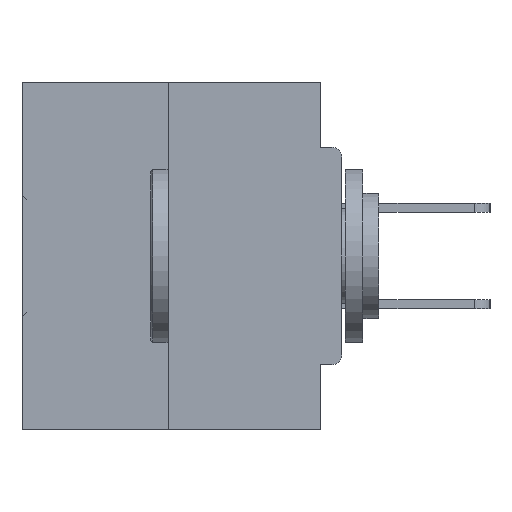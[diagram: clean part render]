
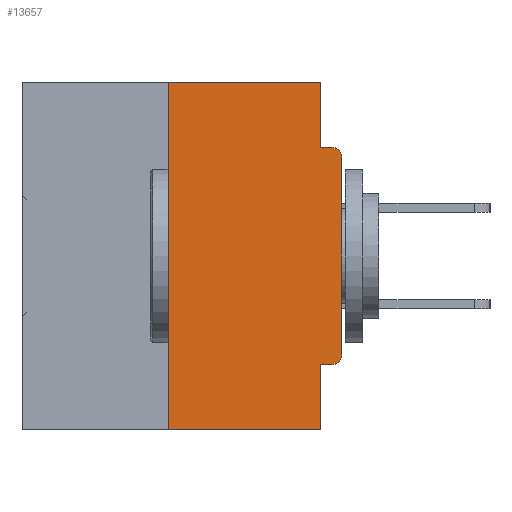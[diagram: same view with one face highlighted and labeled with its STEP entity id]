
A CAD part, left-side view. The second image highlights one B-rep face of the part: STEP entity #13657.
In plain terms, the highlighted planar face has unit normal (-1, 0, 0).
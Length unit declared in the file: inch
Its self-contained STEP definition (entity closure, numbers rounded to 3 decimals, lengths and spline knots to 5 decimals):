
#447 = CARTESIAN_POINT ( 'NONE',  ( 0., 0.015, -0.1085 ) ) ;
#537 = EDGE_CURVE ( 'NONE', #41187, #37084, #8913, .T. ) ;
#1069 = VECTOR ( 'NONE', #31670, 39.37008 ) ;
#1840 = CARTESIAN_POINT ( 'NONE',  ( 0., 0.031, -0.4065 ) ) ;
#3988 = CARTESIAN_POINT ( 'NONE',  ( 0., 0., -0.3915 ) ) ;
#4064 = VERTEX_POINT ( 'NONE', #1840 ) ;
#4535 = VECTOR ( 'NONE', #21475, 39.37008 ) ;
#4632 = CARTESIAN_POINT ( 'NONE',  ( 0., 0.031, 0. ) ) ;
#4937 = DIRECTION ( 'NONE',  ( 0., 0., -1. ) ) ;
#6304 = VERTEX_POINT ( 'NONE', #32371 ) ;
#6608 = ORIENTED_EDGE ( 'NONE', *, *, #36303, .T. ) ;
#6632 = AXIS2_PLACEMENT_3D ( 'NONE', #26175, #19660, #22784 ) ;
#6746 = DIRECTION ( 'NONE',  ( 0., -1., 0. ) ) ;
#7027 = VERTEX_POINT ( 'NONE', #24200 ) ;
#7271 = VECTOR ( 'NONE', #23623, 39.37008 ) ;
#7491 = DIRECTION ( 'NONE',  ( -1., 0., 0. ) ) ;
#7842 = LINE ( 'NONE', #17770, #4535 ) ;
#7940 = ORIENTED_EDGE ( 'NONE', *, *, #32972, .F. ) ;
#8913 = LINE ( 'NONE', #41056, #7271 ) ;
#9235 = VECTOR ( 'NONE', #4937, 39.37008 ) ;
#11164 = ORIENTED_EDGE ( 'NONE', *, *, #537, .F. ) ;
#11357 = EDGE_CURVE ( 'NONE', #4064, #7027, #14936, .T. ) ;
#12130 = LINE ( 'NONE', #26361, #39038 ) ;
#12963 = EDGE_CURVE ( 'NONE', #26523, #42302, #18642, .T. ) ;
#13657 = ADVANCED_FACE ( 'NONE', ( #19707 ), #43288, .F. ) ;
#13735 = CARTESIAN_POINT ( 'NONE',  ( 0., 0.031, 0. ) ) ;
#14194 = LINE ( 'NONE', #4632, #9235 ) ;
#14375 = CARTESIAN_POINT ( 'NONE',  ( 0., 0.46, -0.5 ) ) ;
#14936 = LINE ( 'NONE', #36313, #19318 ) ;
#15106 = ORIENTED_EDGE ( 'NONE', *, *, #38545, .F. ) ;
#15261 = DIRECTION ( 'NONE',  ( 0., 0., -1. ) ) ;
#16286 = EDGE_CURVE ( 'NONE', #37921, #42302, #22758, .T. ) ;
#16679 = ORIENTED_EDGE ( 'NONE', *, *, #24940, .F. ) ;
#17695 = CARTESIAN_POINT ( 'NONE',  ( 0., 0., -0.4065 ) ) ;
#17770 = CARTESIAN_POINT ( 'NONE',  ( 0., 0., 0. ) ) ;
#18613 = DIRECTION ( 'NONE',  ( 1., 0., 0. ) ) ;
#18642 = LINE ( 'NONE', #31029, #40022 ) ;
#18664 = EDGE_LOOP ( 'NONE', ( #11164, #15106, #6608, #20464, #7940, #38362, #26435, #30995, #33911, #16679 ) ) ;
#19185 = CIRCLE ( 'NONE', #6632, 0.015 ) ;
#19318 = VECTOR ( 'NONE', #15261, 39.37008 ) ;
#19660 = DIRECTION ( 'NONE',  ( -1., 0., 0. ) ) ;
#19707 = FACE_OUTER_BOUND ( 'NONE', #18664, .T. ) ;
#20464 = ORIENTED_EDGE ( 'NONE', *, *, #11357, .F. ) ;
#20651 = CARTESIAN_POINT ( 'NONE',  ( 0., 0.25, -0.5 ) ) ;
#21475 = DIRECTION ( 'NONE',  ( 0., 0., 1. ) ) ;
#22758 = CIRCLE ( 'NONE', #41384, 0.015 ) ;
#22784 = DIRECTION ( 'NONE',  ( 0., 0., -1. ) ) ;
#23623 = DIRECTION ( 'NONE',  ( 0., -1., 0. ) ) ;
#24200 = CARTESIAN_POINT ( 'NONE',  ( 0., 0.031, -0.5 ) ) ;
#24855 = DIRECTION ( 'NONE',  ( 0., -1., 0. ) ) ;
#24915 = DIRECTION ( 'NONE',  ( 0., 0., -1. ) ) ;
#24940 = EDGE_CURVE ( 'NONE', #37084, #26523, #14194, .T. ) ;
#25851 = CARTESIAN_POINT ( 'NONE',  ( 0., 0.46, 0. ) ) ;
#26175 = CARTESIAN_POINT ( 'NONE',  ( 0., 0.015, -0.3915 ) ) ;
#26361 = CARTESIAN_POINT ( 'NONE',  ( 0., 0.25, 0. ) ) ;
#26435 = ORIENTED_EDGE ( 'NONE', *, *, #36073, .T. ) ;
#26523 = VERTEX_POINT ( 'NONE', #44175 ) ;
#30957 = CARTESIAN_POINT ( 'NONE',  ( 0., 0.015, -0.0935 ) ) ;
#30995 = ORIENTED_EDGE ( 'NONE', *, *, #16286, .T. ) ;
#31007 = VERTEX_POINT ( 'NONE', #20651 ) ;
#31029 = CARTESIAN_POINT ( 'NONE',  ( 0., 0., -0.0935 ) ) ;
#31291 = LINE ( 'NONE', #17695, #1069 ) ;
#31670 = DIRECTION ( 'NONE',  ( 0., 1., 0. ) ) ;
#32371 = CARTESIAN_POINT ( 'NONE',  ( 0., 0.015, -0.4065 ) ) ;
#32507 = AXIS2_PLACEMENT_3D ( 'NONE', #25851, #18613, #35971 ) ;
#32951 = VERTEX_POINT ( 'NONE', #3988 ) ;
#32972 = EDGE_CURVE ( 'NONE', #6304, #4064, #31291, .T. ) ;
#33211 = EDGE_CURVE ( 'NONE', #6304, #32951, #19185, .T. ) ;
#33911 = ORIENTED_EDGE ( 'NONE', *, *, #12963, .F. ) ;
#34101 = LINE ( 'NONE', #14375, #35162 ) ;
#35162 = VECTOR ( 'NONE', #24855, 39.37008 ) ;
#35971 = DIRECTION ( 'NONE',  ( 0., 0., -1. ) ) ;
#36073 = EDGE_CURVE ( 'NONE', #32951, #37921, #7842, .T. ) ;
#36303 = EDGE_CURVE ( 'NONE', #31007, #7027, #34101, .T. ) ;
#36313 = CARTESIAN_POINT ( 'NONE',  ( 0., 0.031, -0.5 ) ) ;
#36375 = CARTESIAN_POINT ( 'NONE',  ( 0., 0.25, 0. ) ) ;
#37054 = DIRECTION ( 'NONE',  ( 0., 0., 1. ) ) ;
#37084 = VERTEX_POINT ( 'NONE', #13735 ) ;
#37921 = VERTEX_POINT ( 'NONE', #38063 ) ;
#38063 = CARTESIAN_POINT ( 'NONE',  ( 0., 0., -0.1085 ) ) ;
#38362 = ORIENTED_EDGE ( 'NONE', *, *, #33211, .T. ) ;
#38545 = EDGE_CURVE ( 'NONE', #31007, #41187, #12130, .T. ) ;
#39038 = VECTOR ( 'NONE', #37054, 39.37008 ) ;
#40022 = VECTOR ( 'NONE', #6746, 39.37008 ) ;
#41056 = CARTESIAN_POINT ( 'NONE',  ( 0., 0.46, 0. ) ) ;
#41187 = VERTEX_POINT ( 'NONE', #36375 ) ;
#41384 = AXIS2_PLACEMENT_3D ( 'NONE', #447, #7491, #24915 ) ;
#42302 = VERTEX_POINT ( 'NONE', #30957 ) ;
#43288 = PLANE ( 'NONE',  #32507 ) ;
#44175 = CARTESIAN_POINT ( 'NONE',  ( 0., 0.031, -0.0935 ) ) ;
